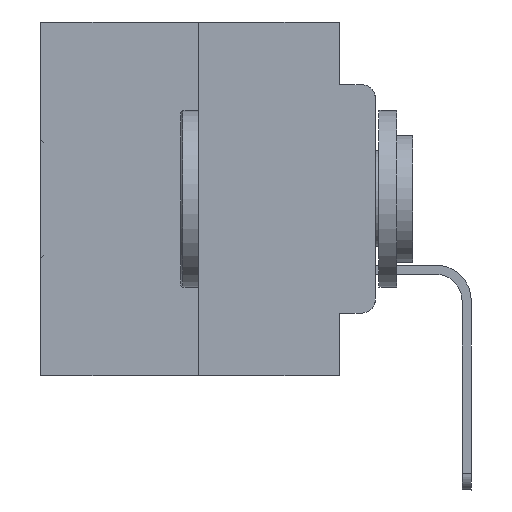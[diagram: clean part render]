
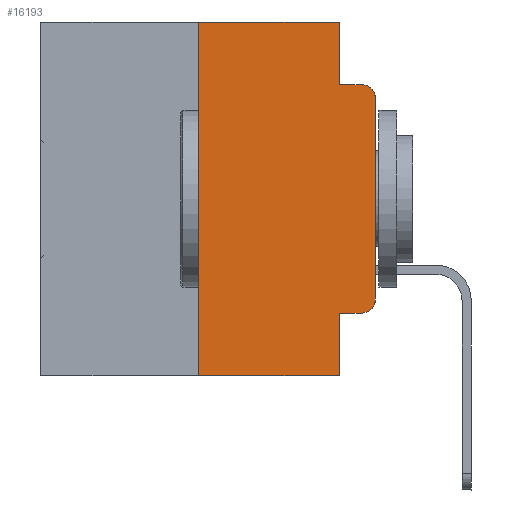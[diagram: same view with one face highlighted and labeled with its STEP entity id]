
A CAD part, left-side view. The second image highlights one B-rep face of the part: STEP entity #16193.
In plain terms, the highlighted planar face has unit normal (-1, 0, 0).
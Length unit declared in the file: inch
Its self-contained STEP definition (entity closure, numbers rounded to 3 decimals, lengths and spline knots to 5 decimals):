
#179 = EDGE_CURVE ( 'NONE', #22837, #14081, #24547, .T. ) ;
#501 = VECTOR ( 'NONE', #13605, 39.37008 ) ;
#1726 = ORIENTED_EDGE ( 'NONE', *, *, #17380, .T. ) ;
#1810 = VECTOR ( 'NONE', #30225, 39.37008 ) ;
#2208 = ORIENTED_EDGE ( 'NONE', *, *, #6862, .T. ) ;
#2291 = DIRECTION ( 'NONE',  ( 0., 0., -1. ) ) ;
#2357 = DIRECTION ( 'NONE',  ( 0., -1., 0. ) ) ;
#2532 = VERTEX_POINT ( 'NONE', #29606 ) ;
#2898 = ORIENTED_EDGE ( 'NONE', *, *, #179, .F. ) ;
#3392 = VERTEX_POINT ( 'NONE', #7272 ) ;
#3421 = CARTESIAN_POINT ( 'NONE',  ( 0., 0.473, 0. ) ) ;
#3652 = ORIENTED_EDGE ( 'NONE', *, *, #21480, .T. ) ;
#3728 = DIRECTION ( 'NONE',  ( 0., 0., -1. ) ) ;
#4420 = LINE ( 'NONE', #19692, #12896 ) ;
#4500 = ORIENTED_EDGE ( 'NONE', *, *, #22674, .F. ) ;
#4885 = DIRECTION ( 'NONE',  ( -1., 0., 0. ) ) ;
#5530 = DIRECTION ( 'NONE',  ( 0., -1., 0. ) ) ;
#5906 = DIRECTION ( 'NONE',  ( 0., 0., 1. ) ) ;
#6862 = EDGE_CURVE ( 'NONE', #30055, #28845, #15338, .T. ) ;
#6905 = ORIENTED_EDGE ( 'NONE', *, *, #7982, .F. ) ;
#7109 = LINE ( 'NONE', #30204, #31515 ) ;
#7272 = CARTESIAN_POINT ( 'NONE',  ( 0., 0.25, 0. ) ) ;
#7542 = VERTEX_POINT ( 'NONE', #24996 ) ;
#7564 = LINE ( 'NONE', #27729, #9484 ) ;
#7591 = EDGE_CURVE ( 'NONE', #28845, #7542, #12187, .T. ) ;
#7982 = EDGE_CURVE ( 'NONE', #2532, #7542, #4420, .T. ) ;
#8138 = DIRECTION ( 'NONE',  ( 0., 0., -1. ) ) ;
#8707 = AXIS2_PLACEMENT_3D ( 'NONE', #27149, #4885, #2291 ) ;
#8918 = EDGE_CURVE ( 'NONE', #22837, #20013, #20983, .T. ) ;
#9484 = VECTOR ( 'NONE', #25355, 39.37008 ) ;
#10308 = ORIENTED_EDGE ( 'NONE', *, *, #23744, .F. ) ;
#10834 = DIRECTION ( 'NONE',  ( 0., 0., -1. ) ) ;
#12069 = CARTESIAN_POINT ( 'NONE',  ( 0., 0.051, 0. ) ) ;
#12187 = CIRCLE ( 'NONE', #17057, 0.02 ) ;
#12199 = AXIS2_PLACEMENT_3D ( 'NONE', #3421, #13629, #3728 ) ;
#12878 = CARTESIAN_POINT ( 'NONE',  ( 0., 0.473, -0.5 ) ) ;
#12896 = VECTOR ( 'NONE', #2357, 39.37008 ) ;
#13605 = DIRECTION ( 'NONE',  ( 0., -1., 0. ) ) ;
#13629 = DIRECTION ( 'NONE',  ( 1., 0., 0. ) ) ;
#14081 = VERTEX_POINT ( 'NONE', #22988 ) ;
#15338 = LINE ( 'NONE', #20432, #1810 ) ;
#15469 = CARTESIAN_POINT ( 'NONE',  ( 0., 0.02, -0.1085 ) ) ;
#16047 = VECTOR ( 'NONE', #8138, 39.37008 ) ;
#16193 = ADVANCED_FACE ( 'NONE', ( #22875 ), #20820, .F. ) ;
#16822 = CARTESIAN_POINT ( 'NONE',  ( 0., 0.051, -0.4115 ) ) ;
#17057 = AXIS2_PLACEMENT_3D ( 'NONE', #15469, #28121, #10834 ) ;
#17380 = EDGE_CURVE ( 'NONE', #20013, #30055, #27980, .T. ) ;
#18237 = CARTESIAN_POINT ( 'NONE',  ( 0., 0.051, -0.4115 ) ) ;
#19692 = CARTESIAN_POINT ( 'NONE',  ( 0., 0.051, -0.0885 ) ) ;
#19709 = ORIENTED_EDGE ( 'NONE', *, *, #31183, .F. ) ;
#20013 = VERTEX_POINT ( 'NONE', #24998 ) ;
#20282 = LINE ( 'NONE', #23535, #29910 ) ;
#20415 = DIRECTION ( 'NONE',  ( 0., 0., -1. ) ) ;
#20432 = CARTESIAN_POINT ( 'NONE',  ( 0., 0., 0. ) ) ;
#20820 = PLANE ( 'NONE',  #12199 ) ;
#20983 = LINE ( 'NONE', #16822, #501 ) ;
#21152 = EDGE_LOOP ( 'NONE', ( #2208, #27252, #6905, #4500, #10308, #19709, #3652, #2898, #30423, #1726 ) ) ;
#21263 = VERTEX_POINT ( 'NONE', #24352 ) ;
#21480 = EDGE_CURVE ( 'NONE', #21263, #14081, #30803, .T. ) ;
#22674 = EDGE_CURVE ( 'NONE', #24906, #2532, #7109, .T. ) ;
#22837 = VERTEX_POINT ( 'NONE', #18237 ) ;
#22875 = FACE_OUTER_BOUND ( 'NONE', #21152, .T. ) ;
#22988 = CARTESIAN_POINT ( 'NONE',  ( 0., 0.051, -0.5 ) ) ;
#23535 = CARTESIAN_POINT ( 'NONE',  ( 0., 0.25, 0. ) ) ;
#23736 = CARTESIAN_POINT ( 'NONE',  ( 0., 0.051, 0. ) ) ;
#23744 = EDGE_CURVE ( 'NONE', #3392, #24906, #7564, .T. ) ;
#24352 = CARTESIAN_POINT ( 'NONE',  ( 0., 0.25, -0.5 ) ) ;
#24547 = LINE ( 'NONE', #23736, #16047 ) ;
#24906 = VERTEX_POINT ( 'NONE', #12069 ) ;
#24996 = CARTESIAN_POINT ( 'NONE',  ( 0., 0.02, -0.0885 ) ) ;
#24998 = CARTESIAN_POINT ( 'NONE',  ( 0., 0.02, -0.4115 ) ) ;
#25355 = DIRECTION ( 'NONE',  ( 0., -1., 0. ) ) ;
#27149 = CARTESIAN_POINT ( 'NONE',  ( 0., 0.02, -0.3915 ) ) ;
#27252 = ORIENTED_EDGE ( 'NONE', *, *, #7591, .T. ) ;
#27280 = CARTESIAN_POINT ( 'NONE',  ( 0., 0., -0.1085 ) ) ;
#27729 = CARTESIAN_POINT ( 'NONE',  ( 0., 0.473, 0. ) ) ;
#27980 = CIRCLE ( 'NONE', #8707, 0.02 ) ;
#28121 = DIRECTION ( 'NONE',  ( -1., 0., 0. ) ) ;
#28845 = VERTEX_POINT ( 'NONE', #27280 ) ;
#28984 = CARTESIAN_POINT ( 'NONE',  ( 0., 0., -0.3915 ) ) ;
#29606 = CARTESIAN_POINT ( 'NONE',  ( 0., 0.051, -0.0885 ) ) ;
#29910 = VECTOR ( 'NONE', #5906, 39.37008 ) ;
#30055 = VERTEX_POINT ( 'NONE', #28984 ) ;
#30204 = CARTESIAN_POINT ( 'NONE',  ( 0., 0.051, 0. ) ) ;
#30225 = DIRECTION ( 'NONE',  ( 0., 0., 1. ) ) ;
#30423 = ORIENTED_EDGE ( 'NONE', *, *, #8918, .T. ) ;
#30803 = LINE ( 'NONE', #12878, #31210 ) ;
#31183 = EDGE_CURVE ( 'NONE', #21263, #3392, #20282, .T. ) ;
#31210 = VECTOR ( 'NONE', #5530, 39.37008 ) ;
#31515 = VECTOR ( 'NONE', #20415, 39.37008 ) ;
